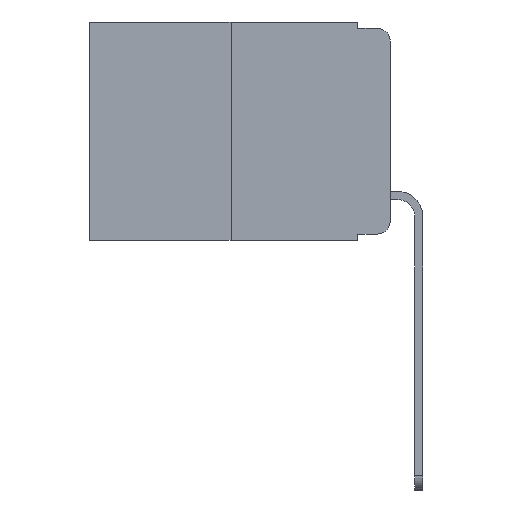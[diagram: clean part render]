
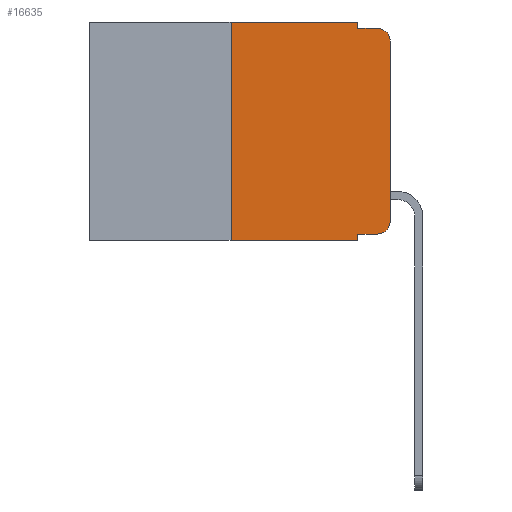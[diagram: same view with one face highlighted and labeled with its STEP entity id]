
A CAD part, left-side view. The second image highlights one B-rep face of the part: STEP entity #16635.
In plain terms, the highlighted planar face has unit normal (-1, 0, 0).
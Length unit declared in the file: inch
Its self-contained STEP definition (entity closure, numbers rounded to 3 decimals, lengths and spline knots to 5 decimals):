
#447 = CARTESIAN_POINT ( 'NONE',  ( 0., 0.051, 0. ) ) ;
#924 = CARTESIAN_POINT ( 'NONE',  ( 0., 0.02, -0.313 ) ) ;
#1171 = CARTESIAN_POINT ( 'NONE',  ( 0., 0.02, -0.333 ) ) ;
#1290 = VERTEX_POINT ( 'NONE', #13636 ) ;
#1703 = LINE ( 'NONE', #447, #6775 ) ;
#3189 = ORIENTED_EDGE ( 'NONE', *, *, #5320, .T. ) ;
#3500 = EDGE_CURVE ( 'NONE', #14256, #11171, #11036, .T. ) ;
#3630 = CARTESIAN_POINT ( 'NONE',  ( 0., 0.02, -0.01 ) ) ;
#3679 = DIRECTION ( 'NONE',  ( 0., 0., 1. ) ) ;
#4443 = DIRECTION ( 'NONE',  ( -1., 0., 0. ) ) ;
#4445 = EDGE_LOOP ( 'NONE', ( #7153, #4646, #10342, #15783, #10878, #5240, #14930, #10273, #3189, #11147 ) ) ;
#4498 = DIRECTION ( 'NONE',  ( 0., -1., 0. ) ) ;
#4513 = CARTESIAN_POINT ( 'NONE',  ( 0., 0.051, -0.333 ) ) ;
#4646 = ORIENTED_EDGE ( 'NONE', *, *, #17136, .T. ) ;
#4896 = VERTEX_POINT ( 'NONE', #4513 ) ;
#5066 = CARTESIAN_POINT ( 'NONE',  ( 0., 0.473, -0.343 ) ) ;
#5104 = DIRECTION ( 'NONE',  ( 0., 0., -1. ) ) ;
#5240 = ORIENTED_EDGE ( 'NONE', *, *, #11115, .F. ) ;
#5320 = EDGE_CURVE ( 'NONE', #4896, #14604, #14487, .T. ) ;
#6092 = CIRCLE ( 'NONE', #13156, 0.02 ) ;
#6610 = EDGE_CURVE ( 'NONE', #1290, #17141, #18622, .T. ) ;
#6663 = CARTESIAN_POINT ( 'NONE',  ( 0., 0.25, 0. ) ) ;
#6775 = VECTOR ( 'NONE', #5104, 39.37008 ) ;
#6933 = CARTESIAN_POINT ( 'NONE',  ( 0., 0.051, 0. ) ) ;
#7153 = ORIENTED_EDGE ( 'NONE', *, *, #3500, .T. ) ;
#7235 = CARTESIAN_POINT ( 'NONE',  ( 0., 0.473, 0. ) ) ;
#7400 = CARTESIAN_POINT ( 'NONE',  ( 0., 0.051, -0.333 ) ) ;
#7501 = AXIS2_PLACEMENT_3D ( 'NONE', #16468, #4443, #7541 ) ;
#7541 = DIRECTION ( 'NONE',  ( 0., 0., -1. ) ) ;
#7710 = VERTEX_POINT ( 'NONE', #16632 ) ;
#7832 = CARTESIAN_POINT ( 'NONE',  ( 0., 0.051, -0.01 ) ) ;
#8569 = VECTOR ( 'NONE', #9749, 39.37008 ) ;
#8798 = CIRCLE ( 'NONE', #7501, 0.02 ) ;
#8970 = VERTEX_POINT ( 'NONE', #6663 ) ;
#9378 = CARTESIAN_POINT ( 'NONE',  ( 0., 0.25, 0. ) ) ;
#9441 = VECTOR ( 'NONE', #15668, 39.37008 ) ;
#9749 = DIRECTION ( 'NONE',  ( 0., -1., 0. ) ) ;
#9792 = DIRECTION ( 'NONE',  ( 0., 0., 1. ) ) ;
#9926 = DIRECTION ( 'NONE',  ( 0., 0., -1. ) ) ;
#10273 = ORIENTED_EDGE ( 'NONE', *, *, #16010, .F. ) ;
#10342 = ORIENTED_EDGE ( 'NONE', *, *, #17861, .F. ) ;
#10352 = CARTESIAN_POINT ( 'NONE',  ( 0., 0.051, -0.01 ) ) ;
#10359 = VECTOR ( 'NONE', #9792, 39.37008 ) ;
#10878 = ORIENTED_EDGE ( 'NONE', *, *, #18343, .F. ) ;
#10987 = DIRECTION ( 'NONE',  ( 1., 0., 0. ) ) ;
#11036 = LINE ( 'NONE', #18688, #10359 ) ;
#11115 = EDGE_CURVE ( 'NONE', #14056, #8970, #17583, .T. ) ;
#11147 = ORIENTED_EDGE ( 'NONE', *, *, #13302, .T. ) ;
#11157 = DIRECTION ( 'NONE',  ( -1., 0., 0. ) ) ;
#11171 = VERTEX_POINT ( 'NONE', #18809 ) ;
#11453 = VECTOR ( 'NONE', #4498, 39.37008 ) ;
#12204 = VERTEX_POINT ( 'NONE', #3630 ) ;
#12480 = PLANE ( 'NONE',  #13479 ) ;
#12716 = LINE ( 'NONE', #7235, #9441 ) ;
#12786 = FACE_OUTER_BOUND ( 'NONE', #4445, .T. ) ;
#13043 = VECTOR ( 'NONE', #9926, 39.37008 ) ;
#13156 = AXIS2_PLACEMENT_3D ( 'NONE', #924, #11157, #18502 ) ;
#13302 = EDGE_CURVE ( 'NONE', #14604, #14256, #6092, .T. ) ;
#13479 = AXIS2_PLACEMENT_3D ( 'NONE', #16856, #10987, #15564 ) ;
#13632 = VECTOR ( 'NONE', #3679, 39.37008 ) ;
#13636 = CARTESIAN_POINT ( 'NONE',  ( 0., 0.051, 0. ) ) ;
#13950 = DIRECTION ( 'NONE',  ( 0., -1., 0. ) ) ;
#14056 = VERTEX_POINT ( 'NONE', #15764 ) ;
#14256 = VERTEX_POINT ( 'NONE', #14840 ) ;
#14487 = LINE ( 'NONE', #7400, #11453 ) ;
#14604 = VERTEX_POINT ( 'NONE', #1171 ) ;
#14840 = CARTESIAN_POINT ( 'NONE',  ( 0., 0., -0.313 ) ) ;
#14930 = ORIENTED_EDGE ( 'NONE', *, *, #17387, .T. ) ;
#15564 = DIRECTION ( 'NONE',  ( 0., 0., -1. ) ) ;
#15668 = DIRECTION ( 'NONE',  ( 0., -1., 0. ) ) ;
#15764 = CARTESIAN_POINT ( 'NONE',  ( 0., 0.25, -0.343 ) ) ;
#15783 = ORIENTED_EDGE ( 'NONE', *, *, #6610, .F. ) ;
#16010 = EDGE_CURVE ( 'NONE', #4896, #7710, #1703, .T. ) ;
#16022 = LINE ( 'NONE', #5066, #8569 ) ;
#16468 = CARTESIAN_POINT ( 'NONE',  ( 0., 0.02, -0.03 ) ) ;
#16474 = VECTOR ( 'NONE', #13950, 39.37008 ) ;
#16632 = CARTESIAN_POINT ( 'NONE',  ( 0., 0.051, -0.343 ) ) ;
#16635 = ADVANCED_FACE ( 'NONE', ( #12786 ), #12480, .F. ) ;
#16856 = CARTESIAN_POINT ( 'NONE',  ( 0., 0.473, 0. ) ) ;
#17136 = EDGE_CURVE ( 'NONE', #11171, #12204, #8798, .T. ) ;
#17141 = VERTEX_POINT ( 'NONE', #10352 ) ;
#17387 = EDGE_CURVE ( 'NONE', #14056, #7710, #16022, .T. ) ;
#17388 = LINE ( 'NONE', #7832, #16474 ) ;
#17583 = LINE ( 'NONE', #9378, #13632 ) ;
#17861 = EDGE_CURVE ( 'NONE', #17141, #12204, #17388, .T. ) ;
#18343 = EDGE_CURVE ( 'NONE', #8970, #1290, #12716, .T. ) ;
#18502 = DIRECTION ( 'NONE',  ( 0., 0., -1. ) ) ;
#18622 = LINE ( 'NONE', #6933, #13043 ) ;
#18688 = CARTESIAN_POINT ( 'NONE',  ( 0., 0., 0. ) ) ;
#18809 = CARTESIAN_POINT ( 'NONE',  ( 0., 0., -0.03 ) ) ;
